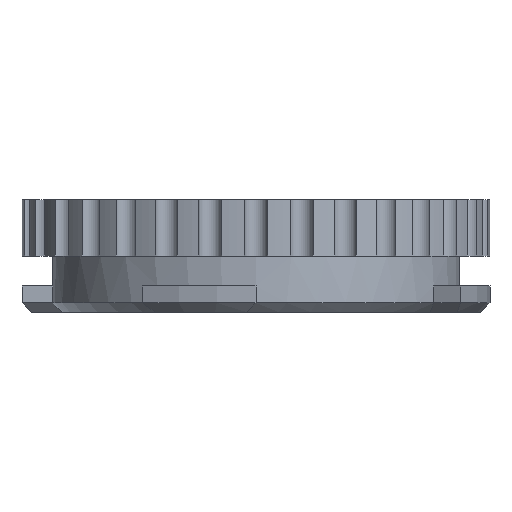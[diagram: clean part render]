
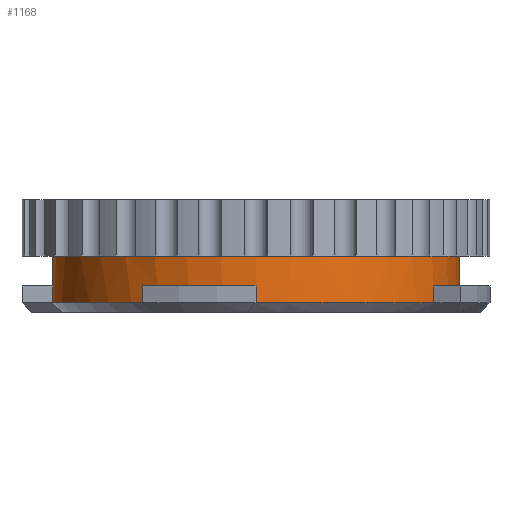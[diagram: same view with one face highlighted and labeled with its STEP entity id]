
A CAD part, front view. The second image highlights one B-rep face of the part: STEP entity #1168.
In plain terms, the highlighted cylindrical face has radius 13.787 mm (diameter 27.575 mm), a partial arc.
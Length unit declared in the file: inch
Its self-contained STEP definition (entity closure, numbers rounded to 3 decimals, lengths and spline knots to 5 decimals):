
#304 = VECTOR ( 'NONE', #5287, 39.37008 ) ;
#427 = LINE ( 'NONE', #7522, #5252 ) ;
#884 = ORIENTED_EDGE ( 'NONE', *, *, #1466, .T. ) ;
#1002 = CARTESIAN_POINT ( 'NONE',  ( -0.54281, 0., 0.15 ) ) ;
#1168 = ADVANCED_FACE ( 'NONE', ( #5362 ), #5351, .T. ) ;
#1201 = EDGE_CURVE ( 'NONE', #7192, #3294, #7215, .T. ) ;
#1210 = ORIENTED_EDGE ( 'NONE', *, *, #6367, .T. ) ;
#1409 = CIRCLE ( 'NONE', #10125, 0.54281 ) ;
#1466 = EDGE_CURVE ( 'NONE', #6563, #3488, #1518, .T. ) ;
#1518 = CIRCLE ( 'NONE', #8258, 0.54281 ) ;
#1658 = CARTESIAN_POINT ( 'NONE',  ( 0., -0.54281, 0.02461 ) ) ;
#1713 = CARTESIAN_POINT ( 'NONE',  ( 0., 0., 0.07 ) ) ;
#1755 = DIRECTION ( 'NONE',  ( 1., 0., 0. ) ) ;
#1786 = EDGE_CURVE ( 'NONE', #6770, #7192, #3856, .T. ) ;
#1893 = CARTESIAN_POINT ( 'NONE',  ( 0., -0.54281, 0.15 ) ) ;
#1899 = VERTEX_POINT ( 'NONE', #6994 ) ;
#1966 = EDGE_CURVE ( 'NONE', #3294, #6563, #2395, .T. ) ;
#2013 = ORIENTED_EDGE ( 'NONE', *, *, #7433, .T. ) ;
#2058 = DIRECTION ( 'NONE',  ( 0., 0., 1. ) ) ;
#2084 = CARTESIAN_POINT ( 'NONE',  ( 0., 0., 0.07 ) ) ;
#2202 = DIRECTION ( 'NONE',  ( 1., 0., 0. ) ) ;
#2220 = CARTESIAN_POINT ( 'NONE',  ( 0., 0., 0.15 ) ) ;
#2246 = VECTOR ( 'NONE', #7430, 39.37008 ) ;
#2395 = LINE ( 'NONE', #6027, #304 ) ;
#2556 = CARTESIAN_POINT ( 'NONE',  ( -0.26316, -0.47476, 0.07 ) ) ;
#2789 = DIRECTION ( 'NONE',  ( 0., 0., 1. ) ) ;
#3187 = VERTEX_POINT ( 'NONE', #2556 ) ;
#3190 = AXIS2_PLACEMENT_3D ( 'NONE', #2220, #3848, #6976 ) ;
#3239 = ORIENTED_EDGE ( 'NONE', *, *, #1786, .T. ) ;
#3253 = CARTESIAN_POINT ( 'NONE',  ( 0., 0., 0.02461 ) ) ;
#3264 = LINE ( 'NONE', #8197, #7365 ) ;
#3294 = VERTEX_POINT ( 'NONE', #4924 ) ;
#3488 = VERTEX_POINT ( 'NONE', #7008 ) ;
#3616 = CARTESIAN_POINT ( 'NONE',  ( -0.54281, 0., 0.02461 ) ) ;
#3787 = CARTESIAN_POINT ( 'NONE',  ( -0.54281, 0., 0.07 ) ) ;
#3848 = DIRECTION ( 'NONE',  ( 0., 0., -1. ) ) ;
#3856 = LINE ( 'NONE', #1893, #2246 ) ;
#3954 = AXIS2_PLACEMENT_3D ( 'NONE', #6164, #4491, #2202 ) ;
#3971 = CIRCLE ( 'NONE', #3954, 0.54281 ) ;
#4068 = AXIS2_PLACEMENT_3D ( 'NONE', #9474, #4578, #4714 ) ;
#4259 = CARTESIAN_POINT ( 'NONE',  ( 0., -0.54281, 0.07 ) ) ;
#4386 = VECTOR ( 'NONE', #5133, 39.37008 ) ;
#4477 = ORIENTED_EDGE ( 'NONE', *, *, #1966, .T. ) ;
#4491 = DIRECTION ( 'NONE',  ( 0., 0., 1. ) ) ;
#4578 = DIRECTION ( 'NONE',  ( 0., 0., 1. ) ) ;
#4714 = DIRECTION ( 'NONE',  ( 1., 0., 0. ) ) ;
#4717 = CARTESIAN_POINT ( 'NONE',  ( 0.47476, -0.26316, 0.07 ) ) ;
#4721 = VERTEX_POINT ( 'NONE', #3616 ) ;
#4779 = EDGE_CURVE ( 'NONE', #4721, #10056, #3971, .T. ) ;
#4924 = CARTESIAN_POINT ( 'NONE',  ( 0.47476, -0.26316, 0.02461 ) ) ;
#4949 = ORIENTED_EDGE ( 'NONE', *, *, #8215, .F. ) ;
#4960 = VERTEX_POINT ( 'NONE', #10035 ) ;
#5021 = DIRECTION ( 'NONE',  ( 0., 0., -1. ) ) ;
#5133 = DIRECTION ( 'NONE',  ( 0., 0., -1. ) ) ;
#5252 = VECTOR ( 'NONE', #2789, 39.37008 ) ;
#5287 = DIRECTION ( 'NONE',  ( 0., 0., 1. ) ) ;
#5351 = CYLINDRICAL_SURFACE ( 'NONE', #3190, 0.54281 ) ;
#5362 = FACE_OUTER_BOUND ( 'NONE', #6565, .T. ) ;
#5591 = ORIENTED_EDGE ( 'NONE', *, *, #1201, .T. ) ;
#5884 = DIRECTION ( 'NONE',  ( 0., 0., -1. ) ) ;
#6027 = CARTESIAN_POINT ( 'NONE',  ( 0.47476, -0.26316, 0.15 ) ) ;
#6028 = VERTEX_POINT ( 'NONE', #3787 ) ;
#6164 = CARTESIAN_POINT ( 'NONE',  ( 0., 0., 0.02461 ) ) ;
#6223 = ORIENTED_EDGE ( 'NONE', *, *, #6371, .T. ) ;
#6235 = ORIENTED_EDGE ( 'NONE', *, *, #7324, .F. ) ;
#6327 = ORIENTED_EDGE ( 'NONE', *, *, #10048, .T. ) ;
#6367 = EDGE_CURVE ( 'NONE', #10056, #3187, #427, .T. ) ;
#6371 = EDGE_CURVE ( 'NONE', #1899, #6028, #7124, .T. ) ;
#6563 = VERTEX_POINT ( 'NONE', #4717 ) ;
#6565 = EDGE_LOOP ( 'NONE', ( #6235, #4949, #6223, #6327, #7937, #1210, #2013, #3239, #5591, #4477, #884 ) ) ;
#6770 = VERTEX_POINT ( 'NONE', #4259 ) ;
#6976 = DIRECTION ( 'NONE',  ( -1., 0., 0. ) ) ;
#6994 = CARTESIAN_POINT ( 'NONE',  ( -0.54281, 0., 0.15 ) ) ;
#7008 = CARTESIAN_POINT ( 'NONE',  ( 0.54281, 0., 0.07 ) ) ;
#7124 = LINE ( 'NONE', #10160, #4386 ) ;
#7163 = DIRECTION ( 'NONE',  ( 0., 0., 1. ) ) ;
#7192 = VERTEX_POINT ( 'NONE', #1658 ) ;
#7215 = CIRCLE ( 'NONE', #7785, 0.54281 ) ;
#7324 = EDGE_CURVE ( 'NONE', #4960, #3488, #3264, .T. ) ;
#7365 = VECTOR ( 'NONE', #5884, 39.37008 ) ;
#7430 = DIRECTION ( 'NONE',  ( 0., 0., -1. ) ) ;
#7433 = EDGE_CURVE ( 'NONE', #3187, #6770, #1409, .T. ) ;
#7522 = CARTESIAN_POINT ( 'NONE',  ( -0.26316, -0.47476, 0.15 ) ) ;
#7556 = LINE ( 'NONE', #1002, #9673 ) ;
#7785 = AXIS2_PLACEMENT_3D ( 'NONE', #3253, #9532, #8711 ) ;
#7937 = ORIENTED_EDGE ( 'NONE', *, *, #4779, .T. ) ;
#8112 = CARTESIAN_POINT ( 'NONE',  ( -0.26316, -0.47476, 0.02461 ) ) ;
#8197 = CARTESIAN_POINT ( 'NONE',  ( 0.54281, 0., 0.15 ) ) ;
#8215 = EDGE_CURVE ( 'NONE', #1899, #4960, #8333, .T. ) ;
#8258 = AXIS2_PLACEMENT_3D ( 'NONE', #1713, #7163, #1755 ) ;
#8294 = DIRECTION ( 'NONE',  ( 0., -1., 0. ) ) ;
#8333 = CIRCLE ( 'NONE', #4068, 0.54281 ) ;
#8711 = DIRECTION ( 'NONE',  ( 1., 0., 0. ) ) ;
#9474 = CARTESIAN_POINT ( 'NONE',  ( 0., 0., 0.15 ) ) ;
#9532 = DIRECTION ( 'NONE',  ( 0., 0., 1. ) ) ;
#9673 = VECTOR ( 'NONE', #5021, 39.37008 ) ;
#10035 = CARTESIAN_POINT ( 'NONE',  ( 0.54281, 0., 0.15 ) ) ;
#10048 = EDGE_CURVE ( 'NONE', #6028, #4721, #7556, .T. ) ;
#10056 = VERTEX_POINT ( 'NONE', #8112 ) ;
#10125 = AXIS2_PLACEMENT_3D ( 'NONE', #2084, #2058, #8294 ) ;
#10160 = CARTESIAN_POINT ( 'NONE',  ( -0.54281, 0., 0.15 ) ) ;
